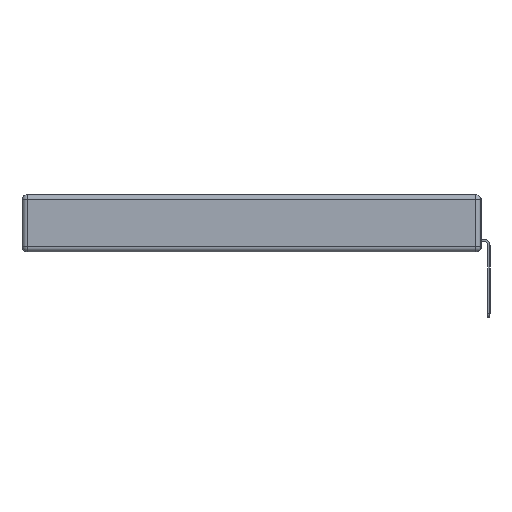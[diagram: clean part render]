
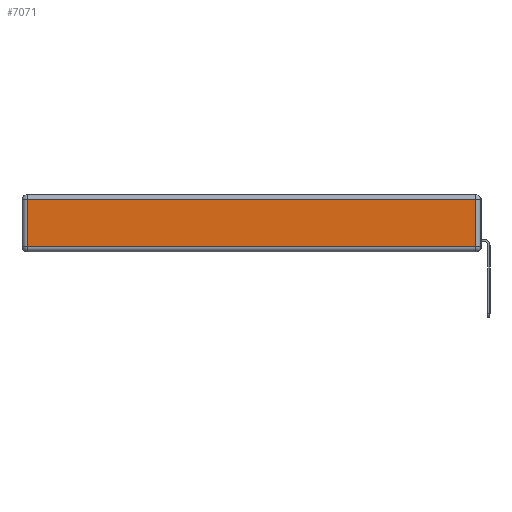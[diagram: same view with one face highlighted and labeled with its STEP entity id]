
A CAD part, left-side view. The second image highlights one B-rep face of the part: STEP entity #7071.
In plain terms, the highlighted planar face has unit normal (-1, 0, 0).
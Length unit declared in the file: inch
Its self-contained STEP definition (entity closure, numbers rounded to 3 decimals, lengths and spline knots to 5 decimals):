
#942 = CARTESIAN_POINT ( 'NONE',  ( 0., 0.03, -0.03 ) ) ;
#1734 = CARTESIAN_POINT ( 'NONE',  ( 0., 2.72, -0.03 ) ) ;
#1808 = CARTESIAN_POINT ( 'NONE',  ( 0., 2.75, -0.03 ) ) ;
#2637 = DIRECTION ( 'NONE',  ( 0., -1., 0. ) ) ;
#2704 = VECTOR ( 'NONE', #2637, 39.37008 ) ;
#2770 = DIRECTION ( 'NONE',  ( 0., 1., 0. ) ) ;
#2814 = DIRECTION ( 'NONE',  ( 0., 0., 1. ) ) ;
#3947 = EDGE_CURVE ( 'NONE', #10913, #13128, #7918, .T. ) ;
#4208 = VERTEX_POINT ( 'NONE', #1734 ) ;
#4555 = CARTESIAN_POINT ( 'NONE',  ( 0., 0.03, -0.343 ) ) ;
#4629 = EDGE_CURVE ( 'NONE', #14595, #10913, #4936, .T. ) ;
#4936 = LINE ( 'NONE', #8531, #2704 ) ;
#5386 = DIRECTION ( 'NONE',  ( 0., 0., 1. ) ) ;
#6016 = PLANE ( 'NONE',  #8455 ) ;
#7056 = LINE ( 'NONE', #7281, #10883 ) ;
#7071 = ADVANCED_FACE ( 'NONE', ( #8402 ), #6016, .T. ) ;
#7174 = CARTESIAN_POINT ( 'NONE',  ( 0., 2.72, -0.313 ) ) ;
#7279 = CARTESIAN_POINT ( 'NONE',  ( 0., 0., -0.343 ) ) ;
#7281 = CARTESIAN_POINT ( 'NONE',  ( 0., 2.72, -0.343 ) ) ;
#7918 = LINE ( 'NONE', #4555, #8165 ) ;
#8098 = CARTESIAN_POINT ( 'NONE',  ( 0., 0.03, -0.313 ) ) ;
#8165 = VECTOR ( 'NONE', #5386, 39.37008 ) ;
#8331 = EDGE_CURVE ( 'NONE', #4208, #14595, #7056, .T. ) ;
#8352 = LINE ( 'NONE', #1808, #10682 ) ;
#8402 = FACE_OUTER_BOUND ( 'NONE', #11275, .T. ) ;
#8455 = AXIS2_PLACEMENT_3D ( 'NONE', #7279, #12988, #2814 ) ;
#8531 = CARTESIAN_POINT ( 'NONE',  ( 0., 0., -0.313 ) ) ;
#10262 = EDGE_CURVE ( 'NONE', #13128, #4208, #8352, .T. ) ;
#10682 = VECTOR ( 'NONE', #2770, 39.37008 ) ;
#10883 = VECTOR ( 'NONE', #11577, 39.37008 ) ;
#10913 = VERTEX_POINT ( 'NONE', #8098 ) ;
#11254 = ORIENTED_EDGE ( 'NONE', *, *, #10262, .T. ) ;
#11275 = EDGE_LOOP ( 'NONE', ( #13791, #14058, #11254, #14498 ) ) ;
#11577 = DIRECTION ( 'NONE',  ( 0., 0., -1. ) ) ;
#12988 = DIRECTION ( 'NONE',  ( -1., 0., 0. ) ) ;
#13128 = VERTEX_POINT ( 'NONE', #942 ) ;
#13791 = ORIENTED_EDGE ( 'NONE', *, *, #4629, .T. ) ;
#14058 = ORIENTED_EDGE ( 'NONE', *, *, #3947, .T. ) ;
#14498 = ORIENTED_EDGE ( 'NONE', *, *, #8331, .T. ) ;
#14595 = VERTEX_POINT ( 'NONE', #7174 ) ;
